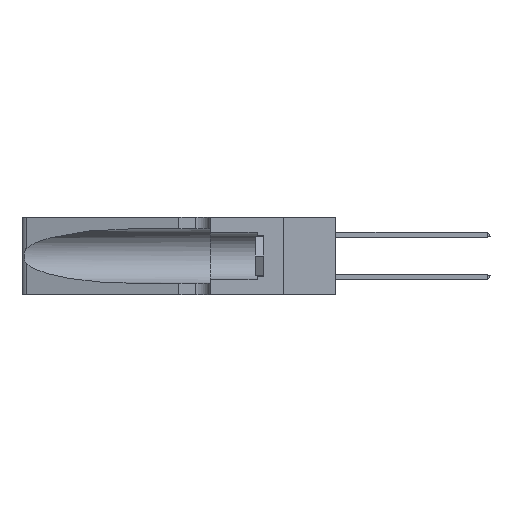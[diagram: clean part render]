
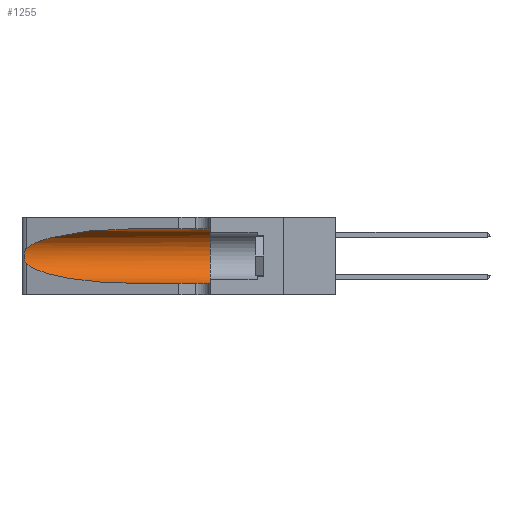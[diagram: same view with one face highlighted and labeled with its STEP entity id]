
A CAD part, left-side view. The second image highlights one B-rep face of the part: STEP entity #1255.
In plain terms, the highlighted cylindrical face has radius 3.308 mm (diameter 6.617 mm), a partial arc.
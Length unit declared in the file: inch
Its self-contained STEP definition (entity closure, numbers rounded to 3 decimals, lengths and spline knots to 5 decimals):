
#187 = VECTOR ( 'NONE', #22980, 39.37008 ) ;
#276 = CARTESIAN_POINT ( 'NONE',  ( 0.1305, 0.35, 0.05475 ) ) ;
#465 = CARTESIAN_POINT ( 'NONE',  ( 0.1305, 0.35, 0.31525 ) ) ;
#921 = AXIS2_PLACEMENT_3D ( 'NONE', #23823, #4623, #6687 ) ;
#1255 = ADVANCED_FACE ( 'NONE', ( #19093 ), #3628, .F. ) ;
#1576 = CARTESIAN_POINT ( 'NONE',  ( 0.25789, 1.23486, 0.15765 ) ) ;
#1866 = CARTESIAN_POINT ( 'NONE',  ( 0.1305, 0.72297, 0.31525 ) ) ;
#2900 = CARTESIAN_POINT ( 'NONE',  ( 0.25487, 1.22718, 0.22369 ) ) ;
#3010 = EDGE_CURVE ( 'NONE', #11508, #18400, #10606, .T. ) ;
#3202 = CARTESIAN_POINT ( 'NONE',  ( 0.25487, 1.22718, 0.14631 ) ) ;
#3511 = EDGE_CURVE ( 'NONE', #22714, #11508, #9368, .T. ) ;
#3622 = CARTESIAN_POINT ( 'NONE',  ( 0.25555, 1.22993, 0.14849 ) ) ;
#3628 = CYLINDRICAL_SURFACE ( 'NONE', #921, 0.13025 ) ;
#3913 = CARTESIAN_POINT ( 'NONE',  ( 0.18966, 0.96281, 0.31525 ) ) ;
#4397 = DIRECTION ( 'NONE',  ( 0., 1., 0. ) ) ;
#4592 = VERTEX_POINT ( 'NONE', #2900 ) ;
#4623 = DIRECTION ( 'NONE',  ( 0., -1., 0. ) ) ;
#4760 = EDGE_CURVE ( 'NONE', #23822, #18516, #9468, .T. ) ;
#4909 = CARTESIAN_POINT ( 'NONE',  ( 0.25487, 1.22718, 0.14631 ) ) ;
#5243 = CARTESIAN_POINT ( 'NONE',  ( 0.1305, 0.72297, 0.05475 ) ) ;
#5563 = CARTESIAN_POINT ( 'NONE',  ( 0.25555, 1.22994, 0.2215 ) ) ;
#5920 = CARTESIAN_POINT ( 'NONE',  ( 0.25487, 1.22718, 0.22369 ) ) ;
#6263 = ORIENTED_EDGE ( 'NONE', *, *, #19398, .T. ) ;
#6687 = DIRECTION ( 'NONE',  ( 0., 0., -1. ) ) ;
#6724 = CARTESIAN_POINT ( 'NONE',  ( 0.1305, 0.72297, 0.05475 ) ) ;
#6888 = EDGE_CURVE ( 'NONE', #4592, #23822, #21024, .T. ) ;
#7254 = ORIENTED_EDGE ( 'NONE', *, *, #3511, .F. ) ;
#7510 = CARTESIAN_POINT ( 'NONE',  ( 0.25787, 1.23484, 0.2124 ) ) ;
#9103 = AXIS2_PLACEMENT_3D ( 'NONE', #16050, #4397, #17949 ) ;
#9172 = ORIENTED_EDGE ( 'NONE', *, *, #6888, .T. ) ;
#9368 = LINE ( 'NONE', #9638, #18416 ) ;
#9447 = CARTESIAN_POINT ( 'NONE',  ( 0.26018, 1.23835, 0.19895 ) ) ;
#9468 =( BOUNDED_CURVE ( )  B_SPLINE_CURVE ( 3, ( #3202, #14920, #16837, #5243 ),
 .UNSPECIFIED., .F., .T. ) 
 B_SPLINE_CURVE_WITH_KNOTS ( ( 4, 4 ),
 ( 3.44316, 4.71239 ),
 .UNSPECIFIED. ) 
 CURVE ( )  GEOMETRIC_REPRESENTATION_ITEM ( )  RATIONAL_B_SPLINE_CURVE ( ( 1., 0.87, 0.87, 1. ) ) 
 REPRESENTATION_ITEM ( '' )  );
#9638 = CARTESIAN_POINT ( 'NONE',  ( 0.1305, 1.61858, 0.31525 ) ) ;
#10236 =( BOUNDED_CURVE ( )  B_SPLINE_CURVE ( 3, ( #1866, #3913, #17496, #5920 ),
 .UNSPECIFIED., .F., .T. ) 
 B_SPLINE_CURVE_WITH_KNOTS ( ( 4, 4 ),
 ( 1.5708, 2.84003 ),
 .UNSPECIFIED. ) 
 CURVE ( )  GEOMETRIC_REPRESENTATION_ITEM ( )  RATIONAL_B_SPLINE_CURVE ( ( 1., 0.87, 0.87, 1. ) ) 
 REPRESENTATION_ITEM ( '' )  );
#10606 = CIRCLE ( 'NONE', #9103, 0.13025 ) ;
#10746 = LINE ( 'NONE', #24902, #187 ) ;
#11401 = CARTESIAN_POINT ( 'NONE',  ( 0.26075, 1.23896, 0.178 ) ) ;
#11508 = VERTEX_POINT ( 'NONE', #465 ) ;
#11605 = DIRECTION ( 'NONE',  ( 0., -1., 0. ) ) ;
#12789 = EDGE_LOOP ( 'NONE', ( #16941, #9172, #20084, #6263, #23692, #7254 ) ) ;
#13372 = CARTESIAN_POINT ( 'NONE',  ( 0.25856, 1.23593, 0.16098 ) ) ;
#14920 = CARTESIAN_POINT ( 'NONE',  ( 0.2373, 1.15595, 0.08982 ) ) ;
#15329 = CARTESIAN_POINT ( 'NONE',  ( 0.25639, 1.23186, 0.15144 ) ) ;
#16004 = CARTESIAN_POINT ( 'NONE',  ( 0.1305, 0.72297, 0.31525 ) ) ;
#16050 = CARTESIAN_POINT ( 'NONE',  ( 0.1305, 0.35, 0.185 ) ) ;
#16837 = CARTESIAN_POINT ( 'NONE',  ( 0.18966, 0.96281, 0.05475 ) ) ;
#16941 = ORIENTED_EDGE ( 'NONE', *, *, #20514, .T. ) ;
#17160 = CARTESIAN_POINT ( 'NONE',  ( 0.25487, 1.22718, 0.22369 ) ) ;
#17243 = CARTESIAN_POINT ( 'NONE',  ( 0.25487, 1.22718, 0.14631 ) ) ;
#17496 = CARTESIAN_POINT ( 'NONE',  ( 0.2373, 1.15595, 0.28018 ) ) ;
#17949 = DIRECTION ( 'NONE',  ( 0., 0., 1. ) ) ;
#18400 = VERTEX_POINT ( 'NONE', #276 ) ;
#18416 = VECTOR ( 'NONE', #11605, 39.37008 ) ;
#18516 = VERTEX_POINT ( 'NONE', #6724 ) ;
#19051 = CARTESIAN_POINT ( 'NONE',  ( 0.25639, 1.23184, 0.21858 ) ) ;
#19093 = FACE_OUTER_BOUND ( 'NONE', #12789, .T. ) ;
#19398 = EDGE_CURVE ( 'NONE', #18516, #18400, #10746, .T. ) ;
#20084 = ORIENTED_EDGE ( 'NONE', *, *, #4760, .T. ) ;
#20514 = EDGE_CURVE ( 'NONE', #22714, #4592, #10236, .T. ) ;
#20966 = CARTESIAN_POINT ( 'NONE',  ( 0.25854, 1.2359, 0.20912 ) ) ;
#21024 = B_SPLINE_CURVE_WITH_KNOTS ( 'NONE', 3,
 ( #17160, #5563, #19051, #7510, #20966, #9447, #22883, #11401, #24823, #13372, #1576, #15329, #3622, #17243 ),
 .UNSPECIFIED., .F., .F.,
 ( 4, 2, 2, 2, 2, 2, 4 ),
 ( 0., 0.00027, 0.00053, 0.00107, 0.0016, 0.00187, 0.00214 ),
 .UNSPECIFIED. ) ;
#22714 = VERTEX_POINT ( 'NONE', #16004 ) ;
#22883 = CARTESIAN_POINT ( 'NONE',  ( 0.26075, 1.23896, 0.19203 ) ) ;
#22980 = DIRECTION ( 'NONE',  ( 0., -1., 0. ) ) ;
#23692 = ORIENTED_EDGE ( 'NONE', *, *, #3010, .F. ) ;
#23822 = VERTEX_POINT ( 'NONE', #4909 ) ;
#23823 = CARTESIAN_POINT ( 'NONE',  ( 0.1305, 1.61858, 0.185 ) ) ;
#24823 = CARTESIAN_POINT ( 'NONE',  ( 0.26017, 1.23833, 0.17102 ) ) ;
#24902 = CARTESIAN_POINT ( 'NONE',  ( 0.1305, 1.61858, 0.05475 ) ) ;
